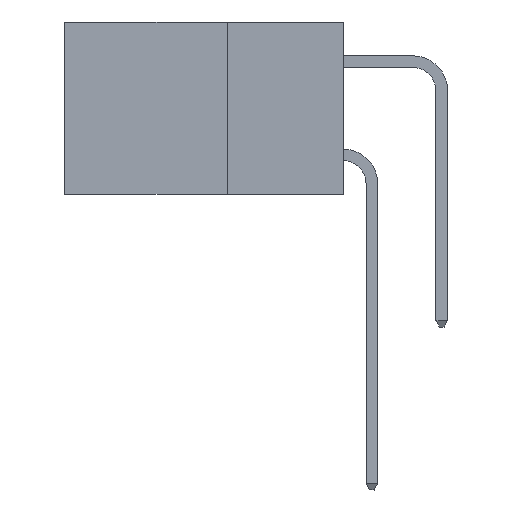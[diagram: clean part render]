
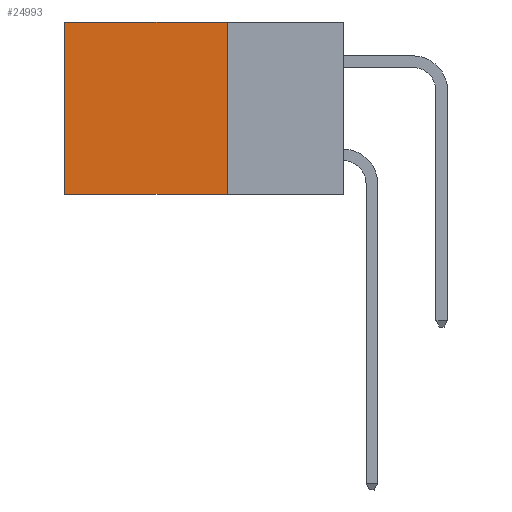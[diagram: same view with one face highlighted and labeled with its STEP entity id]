
A CAD part, left-side view. The second image highlights one B-rep face of the part: STEP entity #24993.
In plain terms, the highlighted planar face has unit normal (-1, 0, 0).
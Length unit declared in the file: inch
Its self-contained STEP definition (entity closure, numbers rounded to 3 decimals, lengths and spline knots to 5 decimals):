
#779 = LINE ( 'NONE', #21345, #5267 ) ;
#1812 = FACE_OUTER_BOUND ( 'NONE', #2172, .T. ) ;
#2172 = EDGE_LOOP ( 'NONE', ( #21797, #8910, #6570, #9917 ) ) ;
#2836 = VECTOR ( 'NONE', #22150, 39.37008 ) ;
#3263 = LINE ( 'NONE', #25828, #13543 ) ;
#5267 = VECTOR ( 'NONE', #6219, 39.37008 ) ;
#6219 = DIRECTION ( 'NONE',  ( 0., 1., 0. ) ) ;
#6570 = ORIENTED_EDGE ( 'NONE', *, *, #23686, .F. ) ;
#7034 = VERTEX_POINT ( 'NONE', #13991 ) ;
#8583 = DIRECTION ( 'NONE',  ( 0., 0., -1. ) ) ;
#8910 = ORIENTED_EDGE ( 'NONE', *, *, #25178, .F. ) ;
#9496 = VERTEX_POINT ( 'NONE', #12032 ) ;
#9917 = ORIENTED_EDGE ( 'NONE', *, *, #11117, .T. ) ;
#9938 = LINE ( 'NONE', #21528, #10624 ) ;
#10624 = VECTOR ( 'NONE', #8583, 39.37008 ) ;
#11117 = EDGE_CURVE ( 'NONE', #25317, #9496, #779, .T. ) ;
#12032 = CARTESIAN_POINT ( 'NONE',  ( 0.298, 0.6, 0. ) ) ;
#12940 = PLANE ( 'NONE',  #21672 ) ;
#13515 = CARTESIAN_POINT ( 'NONE',  ( 0.298, 0.25, -0.37 ) ) ;
#13543 = VECTOR ( 'NONE', #17359, 39.37008 ) ;
#13991 = CARTESIAN_POINT ( 'NONE',  ( 0.298, 0.25, -0.37 ) ) ;
#15113 = DIRECTION ( 'NONE',  ( 0., 0., -1. ) ) ;
#17359 = DIRECTION ( 'NONE',  ( 0., 0., -1. ) ) ;
#18187 = CARTESIAN_POINT ( 'NONE',  ( 0.298, 0.25, 0. ) ) ;
#20259 = EDGE_CURVE ( 'NONE', #9496, #27870, #9938, .T. ) ;
#21345 = CARTESIAN_POINT ( 'NONE',  ( 0.298, 0.25, 0. ) ) ;
#21528 = CARTESIAN_POINT ( 'NONE',  ( 0.298, 0.6, 0. ) ) ;
#21672 = AXIS2_PLACEMENT_3D ( 'NONE', #25724, #27767, #15113 ) ;
#21797 = ORIENTED_EDGE ( 'NONE', *, *, #20259, .T. ) ;
#22150 = DIRECTION ( 'NONE',  ( 0., 1., 0. ) ) ;
#23686 = EDGE_CURVE ( 'NONE', #25317, #7034, #3263, .T. ) ;
#24993 = ADVANCED_FACE ( 'NONE', ( #1812 ), #12940, .F. ) ;
#25178 = EDGE_CURVE ( 'NONE', #7034, #27870, #26428, .T. ) ;
#25317 = VERTEX_POINT ( 'NONE', #18187 ) ;
#25724 = CARTESIAN_POINT ( 'NONE',  ( 0.298, 0.25, 0. ) ) ;
#25828 = CARTESIAN_POINT ( 'NONE',  ( 0.298, 0.25, 0. ) ) ;
#26428 = LINE ( 'NONE', #13515, #2836 ) ;
#26938 = CARTESIAN_POINT ( 'NONE',  ( 0.298, 0.6, -0.37 ) ) ;
#27767 = DIRECTION ( 'NONE',  ( 1., 0., 0. ) ) ;
#27870 = VERTEX_POINT ( 'NONE', #26938 ) ;
